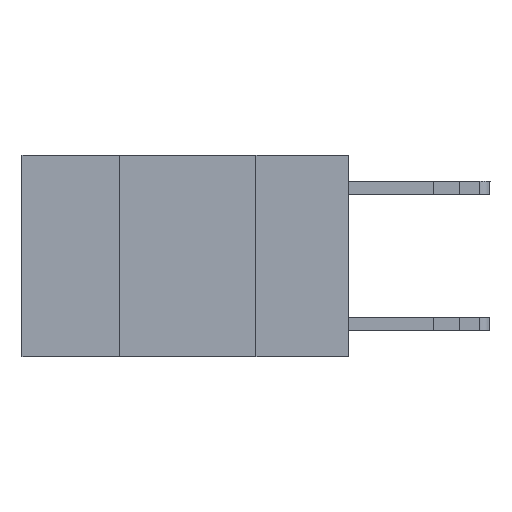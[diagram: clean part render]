
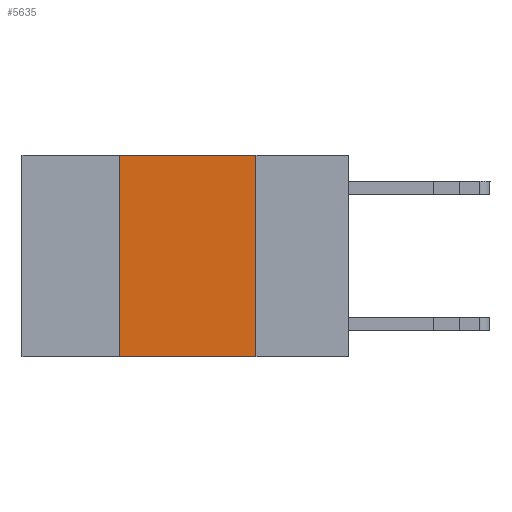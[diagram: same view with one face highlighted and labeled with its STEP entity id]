
A CAD part, left-side view. The second image highlights one B-rep face of the part: STEP entity #5635.
In plain terms, the highlighted planar face has unit normal (-1, 0, 0).
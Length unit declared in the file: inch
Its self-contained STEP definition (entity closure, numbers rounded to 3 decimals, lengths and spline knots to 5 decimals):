
#79 = LINE ( 'NONE', #7311, #15924 ) ;
#293 = DIRECTION ( 'NONE',  ( 0., 0., -1. ) ) ;
#737 = LINE ( 'NONE', #9812, #12486 ) ;
#1360 = DIRECTION ( 'NONE',  ( 0., 0., -1. ) ) ;
#1461 = CARTESIAN_POINT ( 'NONE',  ( 0., 0.6, 0. ) ) ;
#1834 = EDGE_CURVE ( 'NONE', #13849, #18031, #17087, .T. ) ;
#2491 = DIRECTION ( 'NONE',  ( 0., -1., 0. ) ) ;
#3472 = LINE ( 'NONE', #6203, #7104 ) ;
#4042 = VERTEX_POINT ( 'NONE', #12325 ) ;
#5105 = ORIENTED_EDGE ( 'NONE', *, *, #9569, .F. ) ;
#5635 = ADVANCED_FACE ( 'NONE', ( #13495 ), #14869, .F. ) ;
#6103 = DIRECTION ( 'NONE',  ( 0., 0., 1. ) ) ;
#6203 = CARTESIAN_POINT ( 'NONE',  ( 0., 0.42, 0. ) ) ;
#6486 = CARTESIAN_POINT ( 'NONE',  ( 0., 0.6, -0.37 ) ) ;
#6832 = ORIENTED_EDGE ( 'NONE', *, *, #1834, .T. ) ;
#7104 = VECTOR ( 'NONE', #6103, 39.37008 ) ;
#7311 = CARTESIAN_POINT ( 'NONE',  ( 0., 0.17, 0. ) ) ;
#7325 = EDGE_LOOP ( 'NONE', ( #10373, #17387, #5105, #6832 ) ) ;
#7474 = CARTESIAN_POINT ( 'NONE',  ( 0., 0.42, 0. ) ) ;
#9569 = EDGE_CURVE ( 'NONE', #13849, #10787, #3472, .T. ) ;
#9608 = DIRECTION ( 'NONE',  ( 0., -1., 0. ) ) ;
#9812 = CARTESIAN_POINT ( 'NONE',  ( 0., 0.6, 0. ) ) ;
#10373 = ORIENTED_EDGE ( 'NONE', *, *, #11829, .F. ) ;
#10787 = VERTEX_POINT ( 'NONE', #7474 ) ;
#11829 = EDGE_CURVE ( 'NONE', #4042, #18031, #79, .T. ) ;
#12106 = CARTESIAN_POINT ( 'NONE',  ( 0., 0.42, -0.37 ) ) ;
#12325 = CARTESIAN_POINT ( 'NONE',  ( 0., 0.17, 0. ) ) ;
#12486 = VECTOR ( 'NONE', #2491, 39.37008 ) ;
#12544 = EDGE_CURVE ( 'NONE', #10787, #4042, #737, .T. ) ;
#13495 = FACE_OUTER_BOUND ( 'NONE', #7325, .T. ) ;
#13849 = VERTEX_POINT ( 'NONE', #12106 ) ;
#13963 = DIRECTION ( 'NONE',  ( 1., 0., 0. ) ) ;
#14869 = PLANE ( 'NONE',  #15929 ) ;
#15924 = VECTOR ( 'NONE', #1360, 39.37008 ) ;
#15929 = AXIS2_PLACEMENT_3D ( 'NONE', #1461, #13963, #293 ) ;
#16751 = VECTOR ( 'NONE', #9608, 39.37008 ) ;
#17087 = LINE ( 'NONE', #6486, #16751 ) ;
#17279 = CARTESIAN_POINT ( 'NONE',  ( 0., 0.17, -0.37 ) ) ;
#17387 = ORIENTED_EDGE ( 'NONE', *, *, #12544, .F. ) ;
#18031 = VERTEX_POINT ( 'NONE', #17279 ) ;
